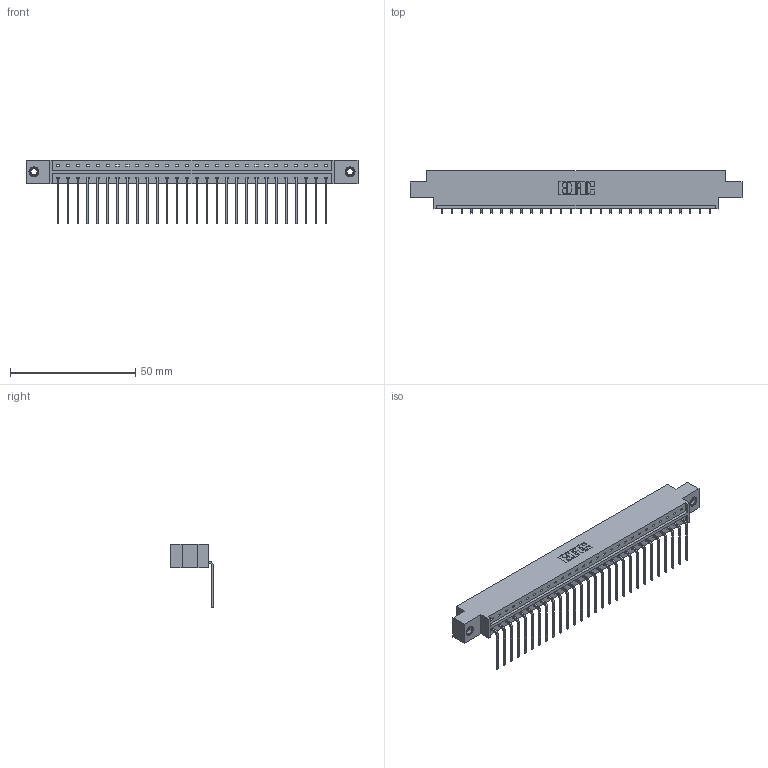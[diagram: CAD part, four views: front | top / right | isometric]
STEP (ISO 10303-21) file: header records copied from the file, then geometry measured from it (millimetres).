
FILE_DESCRIPTION (( 'STEP AP203' ), '1' );
FILE_NAME ('833-028-559-607.STEP', '2020-06-02T10:05:47', ( '' ), ( '' ), 'SwSTEP 2.0', 'SolidWorks 2020', '' );
FILE_SCHEMA (( 'CONFIG_CONTROL_DESIGN' ));
Length unit declared in the file: inch
Products named in the file (4): 833 Part_Offset - .156 Dia - TI; 833-028-559-607; 345-292-001_558 559 Tail - 1; 345-250-001_345-250-005-103
Assembly tree (31 placements, depth 2):
  833-028-559-607
    833 Part_Offset - .156 Dia - TI
    345-292-001_558 559 Tail - 1  x28
    345-250-001_345-250-005-103  x2
Bounding box: 132.49 x 17.09 x 25.53 mm (x, y, z)
Volume: 13063.4 mm3; surface area: 14850.4 mm2
Topology: 31 solids, 31 shells, 1858 faces, 5555 edges, 3658 vertices
Faces by surface type: plane 1338, cylinder 504, cone 12, torus 4
Entity records: 20330 total; most frequent: CARTESIAN_POINT 3493, ORIENTED_EDGE 3450, DIRECTION 3007, EDGE_CURVE 1725, VECTOR 1577, LINE 1577, VERTEX_POINT 1144, AXIS2_PLACEMENT_3D 715
